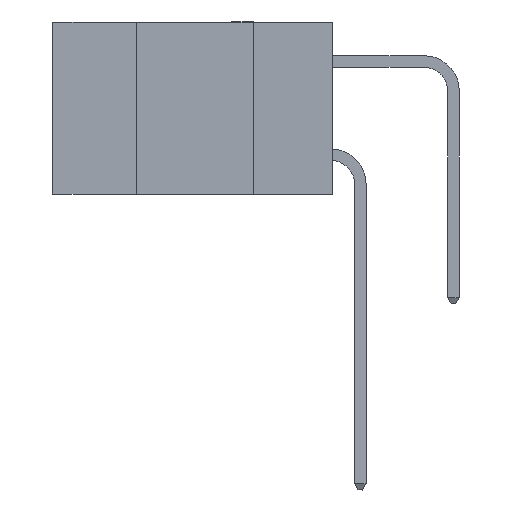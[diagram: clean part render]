
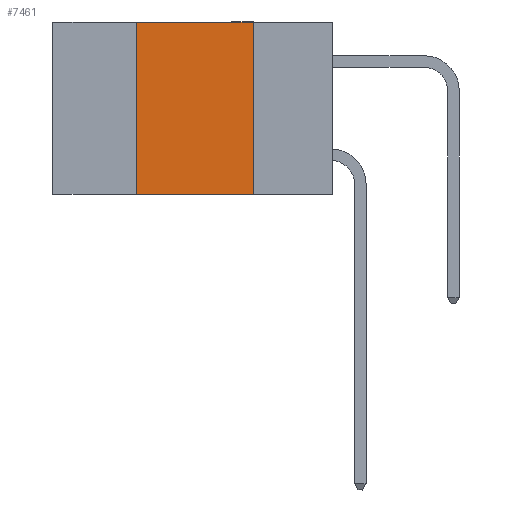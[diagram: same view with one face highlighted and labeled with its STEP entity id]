
A CAD part, left-side view. The second image highlights one B-rep face of the part: STEP entity #7461.
In plain terms, the highlighted planar face has unit normal (-1, 0, 0).
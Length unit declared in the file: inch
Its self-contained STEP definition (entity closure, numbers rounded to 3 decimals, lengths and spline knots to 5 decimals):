
#218 = CARTESIAN_POINT ( 'NONE',  ( 0., 0.17, -0.37 ) ) ;
#915 = LINE ( 'NONE', #11096, #15452 ) ;
#1232 = CARTESIAN_POINT ( 'NONE',  ( 0., 0.6, 0. ) ) ;
#2511 = LINE ( 'NONE', #9637, #13989 ) ;
#3086 = VECTOR ( 'NONE', #11991, 39.37008 ) ;
#3307 = ORIENTED_EDGE ( 'NONE', *, *, #5211, .T. ) ;
#3418 = CARTESIAN_POINT ( 'NONE',  ( 0., 0.6, -0.37 ) ) ;
#3693 = CARTESIAN_POINT ( 'NONE',  ( 0., 0.42, 0. ) ) ;
#3763 = DIRECTION ( 'NONE',  ( 1., 0., 0. ) ) ;
#3786 = VERTEX_POINT ( 'NONE', #218 ) ;
#4517 = AXIS2_PLACEMENT_3D ( 'NONE', #1232, #3763, #14543 ) ;
#4549 = VERTEX_POINT ( 'NONE', #3693 ) ;
#4600 = DIRECTION ( 'NONE',  ( 0., -1., 0. ) ) ;
#4751 = CARTESIAN_POINT ( 'NONE',  ( 0., 0.6, 0. ) ) ;
#4841 = CARTESIAN_POINT ( 'NONE',  ( 0., 0.42, -0.37 ) ) ;
#5030 = DIRECTION ( 'NONE',  ( 0., 0., -1. ) ) ;
#5164 = EDGE_CURVE ( 'NONE', #4549, #9700, #7416, .T. ) ;
#5211 = EDGE_CURVE ( 'NONE', #6743, #3786, #6472, .T. ) ;
#6472 = LINE ( 'NONE', #3418, #10408 ) ;
#6743 = VERTEX_POINT ( 'NONE', #4841 ) ;
#7416 = LINE ( 'NONE', #4751, #3086 ) ;
#7461 = ADVANCED_FACE ( 'NONE', ( #15128 ), #9608, .F. ) ;
#7515 = EDGE_LOOP ( 'NONE', ( #15524, #15619, #11497, #3307 ) ) ;
#7721 = EDGE_CURVE ( 'NONE', #6743, #4549, #2511, .T. ) ;
#8775 = CARTESIAN_POINT ( 'NONE',  ( 0., 0.17, 0. ) ) ;
#9569 = EDGE_CURVE ( 'NONE', #9700, #3786, #915, .T. ) ;
#9608 = PLANE ( 'NONE',  #4517 ) ;
#9637 = CARTESIAN_POINT ( 'NONE',  ( 0., 0.42, 0. ) ) ;
#9700 = VERTEX_POINT ( 'NONE', #8775 ) ;
#10408 = VECTOR ( 'NONE', #4600, 39.37008 ) ;
#11096 = CARTESIAN_POINT ( 'NONE',  ( 0., 0.17, 0. ) ) ;
#11360 = DIRECTION ( 'NONE',  ( 0., 0., 1. ) ) ;
#11497 = ORIENTED_EDGE ( 'NONE', *, *, #7721, .F. ) ;
#11991 = DIRECTION ( 'NONE',  ( 0., -1., 0. ) ) ;
#13989 = VECTOR ( 'NONE', #11360, 39.37008 ) ;
#14543 = DIRECTION ( 'NONE',  ( 0., 0., -1. ) ) ;
#15128 = FACE_OUTER_BOUND ( 'NONE', #7515, .T. ) ;
#15452 = VECTOR ( 'NONE', #5030, 39.37008 ) ;
#15524 = ORIENTED_EDGE ( 'NONE', *, *, #9569, .F. ) ;
#15619 = ORIENTED_EDGE ( 'NONE', *, *, #5164, .F. ) ;
